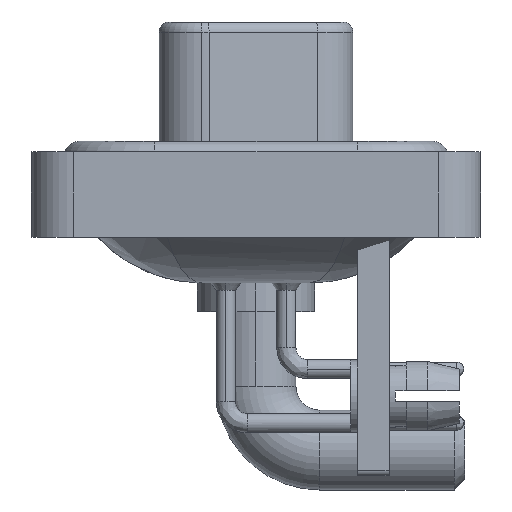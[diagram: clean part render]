
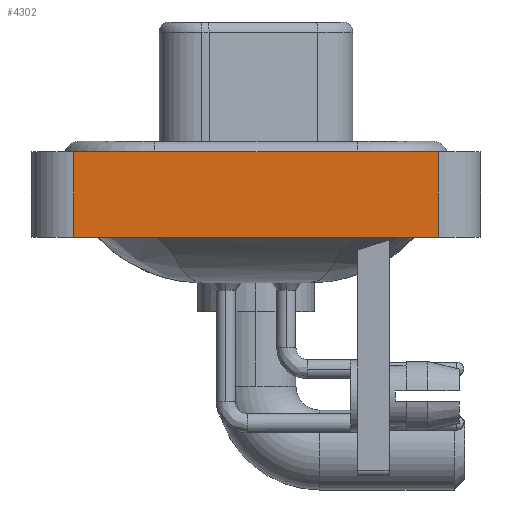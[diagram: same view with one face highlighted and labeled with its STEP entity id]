
A CAD part, left-side view. The second image highlights one B-rep face of the part: STEP entity #4302.
In plain terms, the highlighted planar face has unit normal (-1, 0, 0).
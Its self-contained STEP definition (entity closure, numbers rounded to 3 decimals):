
#405 = DIRECTION ( 'NONE',  ( 0., 0., 1. ) ) ;
#569 = DIRECTION ( 'NONE',  ( 0., -1., 0. ) ) ;
#990 = ORIENTED_EDGE ( 'NONE', *, *, #20509, .F. ) ;
#1118 = DIRECTION ( 'NONE',  ( 0., -1., 0. ) ) ;
#2888 = LINE ( 'NONE', #20774, #12459 ) ;
#3195 = EDGE_LOOP ( 'NONE', ( #6906, #22139, #990, #14075 ) ) ;
#4302 = ADVANCED_FACE ( 'NONE', ( #11694 ), #13619, .T. ) ;
#5006 = AXIS2_PLACEMENT_3D ( 'NONE', #5587, #7628, #25264 ) ;
#5167 = CARTESIAN_POINT ( 'NONE',  ( -7.25, -8.55, -3.6 ) ) ;
#5587 = CARTESIAN_POINT ( 'NONE',  ( -7.25, -8.55, -3.6 ) ) ;
#6906 = ORIENTED_EDGE ( 'NONE', *, *, #15296, .T. ) ;
#7628 = DIRECTION ( 'NONE',  ( -1., 0., 0. ) ) ;
#7910 = VERTEX_POINT ( 'NONE', #5167 ) ;
#9379 = LINE ( 'NONE', #11550, #20665 ) ;
#10243 = CARTESIAN_POINT ( 'NONE',  ( -7.25, -8.55, -3.6 ) ) ;
#11392 = EDGE_CURVE ( 'NONE', #17678, #18359, #2888, .T. ) ;
#11550 = CARTESIAN_POINT ( 'NONE',  ( -7.25, 8.55, -3.6 ) ) ;
#11694 = FACE_OUTER_BOUND ( 'NONE', #3195, .T. ) ;
#12459 = VECTOR ( 'NONE', #1118, 1000. ) ;
#13591 = CARTESIAN_POINT ( 'NONE',  ( -7.25, 8.55, -3.6 ) ) ;
#13619 = PLANE ( 'NONE',  #5006 ) ;
#14043 = CARTESIAN_POINT ( 'NONE',  ( -7.25, -8.55, -3.6 ) ) ;
#14075 = ORIENTED_EDGE ( 'NONE', *, *, #16674, .T. ) ;
#15296 = EDGE_CURVE ( 'NONE', #7910, #18359, #23034, .T. ) ;
#16121 = LINE ( 'NONE', #10243, #16616 ) ;
#16281 = CARTESIAN_POINT ( 'NONE',  ( -7.25, 8.55, 0.4 ) ) ;
#16616 = VECTOR ( 'NONE', #569, 1000. ) ;
#16674 = EDGE_CURVE ( 'NONE', #18032, #7910, #16121, .T. ) ;
#17678 = VERTEX_POINT ( 'NONE', #16281 ) ;
#18032 = VERTEX_POINT ( 'NONE', #13591 ) ;
#18359 = VERTEX_POINT ( 'NONE', #19452 ) ;
#19452 = CARTESIAN_POINT ( 'NONE',  ( -7.25, -8.55, 0.4 ) ) ;
#20509 = EDGE_CURVE ( 'NONE', #18032, #17678, #9379, .T. ) ;
#20665 = VECTOR ( 'NONE', #24858, 1000. ) ;
#20774 = CARTESIAN_POINT ( 'NONE',  ( -7.25, -8.55, 0.4 ) ) ;
#22139 = ORIENTED_EDGE ( 'NONE', *, *, #11392, .F. ) ;
#23034 = LINE ( 'NONE', #14043, #25124 ) ;
#24858 = DIRECTION ( 'NONE',  ( 0., 0., 1. ) ) ;
#25124 = VECTOR ( 'NONE', #405, 1000. ) ;
#25264 = DIRECTION ( 'NONE',  ( 0., 0., 1. ) ) ;
